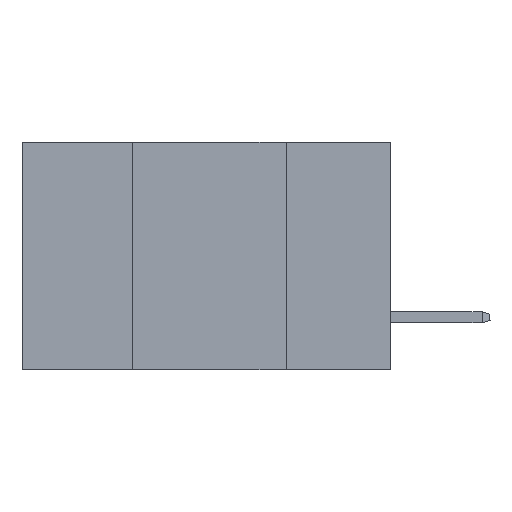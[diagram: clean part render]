
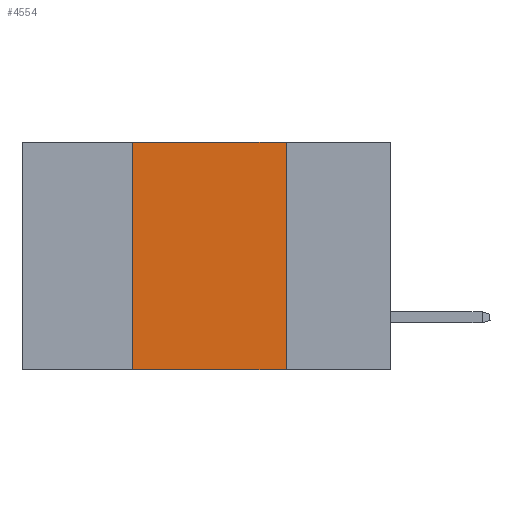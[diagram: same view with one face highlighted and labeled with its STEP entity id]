
A CAD part, left-side view. The second image highlights one B-rep face of the part: STEP entity #4554.
In plain terms, the highlighted planar face has unit normal (-1, 0, 0).
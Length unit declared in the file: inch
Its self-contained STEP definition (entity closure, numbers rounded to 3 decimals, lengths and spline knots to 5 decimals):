
#226 = LINE ( 'NONE', #1112, #8126 ) ;
#756 = CARTESIAN_POINT ( 'NONE',  ( 0., 0.17, -0.37 ) ) ;
#927 = PLANE ( 'NONE',  #13351 ) ;
#1112 = CARTESIAN_POINT ( 'NONE',  ( 0., 0.6, 0. ) ) ;
#1157 = EDGE_CURVE ( 'NONE', #3040, #1993, #8858, .T. ) ;
#1228 = ORIENTED_EDGE ( 'NONE', *, *, #13658, .F. ) ;
#1993 = VERTEX_POINT ( 'NONE', #756 ) ;
#2765 = CARTESIAN_POINT ( 'NONE',  ( 0., 0.17, 0. ) ) ;
#3040 = VERTEX_POINT ( 'NONE', #16616 ) ;
#4287 = CARTESIAN_POINT ( 'NONE',  ( 0., 0.6, 0. ) ) ;
#4449 = CARTESIAN_POINT ( 'NONE',  ( 0., 0.17, 0. ) ) ;
#4554 = ADVANCED_FACE ( 'NONE', ( #8437 ), #927, .F. ) ;
#5376 = VECTOR ( 'NONE', #15102, 39.37008 ) ;
#6579 = VECTOR ( 'NONE', #10905, 39.37008 ) ;
#7640 = ORIENTED_EDGE ( 'NONE', *, *, #10057, .F. ) ;
#7927 = DIRECTION ( 'NONE',  ( 0., -1., 0. ) ) ;
#8126 = VECTOR ( 'NONE', #7927, 39.37008 ) ;
#8287 = ORIENTED_EDGE ( 'NONE', *, *, #1157, .T. ) ;
#8437 = FACE_OUTER_BOUND ( 'NONE', #12811, .T. ) ;
#8858 = LINE ( 'NONE', #10189, #5376 ) ;
#9762 = DIRECTION ( 'NONE',  ( 0., 0., -1. ) ) ;
#10057 = EDGE_CURVE ( 'NONE', #3040, #15109, #11190, .T. ) ;
#10189 = CARTESIAN_POINT ( 'NONE',  ( 0., 0.6, -0.37 ) ) ;
#10905 = DIRECTION ( 'NONE',  ( 0., 0., 1. ) ) ;
#11190 = LINE ( 'NONE', #19529, #6579 ) ;
#12231 = VERTEX_POINT ( 'NONE', #4449 ) ;
#12811 = EDGE_LOOP ( 'NONE', ( #1228, #16873, #7640, #8287 ) ) ;
#12931 = DIRECTION ( 'NONE',  ( 1., 0., 0. ) ) ;
#13159 = EDGE_CURVE ( 'NONE', #15109, #12231, #226, .T. ) ;
#13232 = DIRECTION ( 'NONE',  ( 0., 0., -1. ) ) ;
#13351 = AXIS2_PLACEMENT_3D ( 'NONE', #4287, #12931, #13232 ) ;
#13658 = EDGE_CURVE ( 'NONE', #12231, #1993, #15747, .T. ) ;
#15102 = DIRECTION ( 'NONE',  ( 0., -1., 0. ) ) ;
#15109 = VERTEX_POINT ( 'NONE', #17828 ) ;
#15747 = LINE ( 'NONE', #2765, #16308 ) ;
#16308 = VECTOR ( 'NONE', #9762, 39.37008 ) ;
#16616 = CARTESIAN_POINT ( 'NONE',  ( 0., 0.42, -0.37 ) ) ;
#16873 = ORIENTED_EDGE ( 'NONE', *, *, #13159, .F. ) ;
#17828 = CARTESIAN_POINT ( 'NONE',  ( 0., 0.42, 0. ) ) ;
#19529 = CARTESIAN_POINT ( 'NONE',  ( 0., 0.42, 0. ) ) ;
